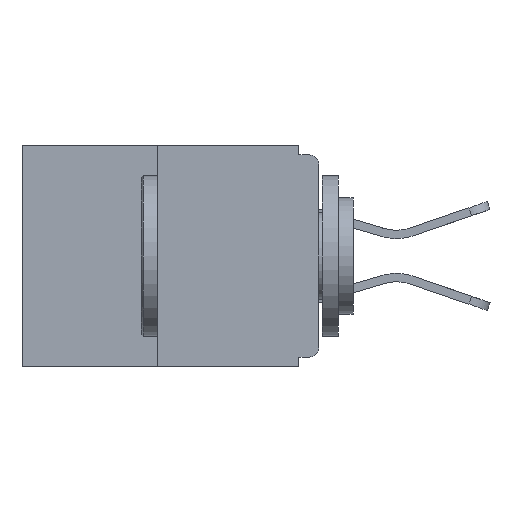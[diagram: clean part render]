
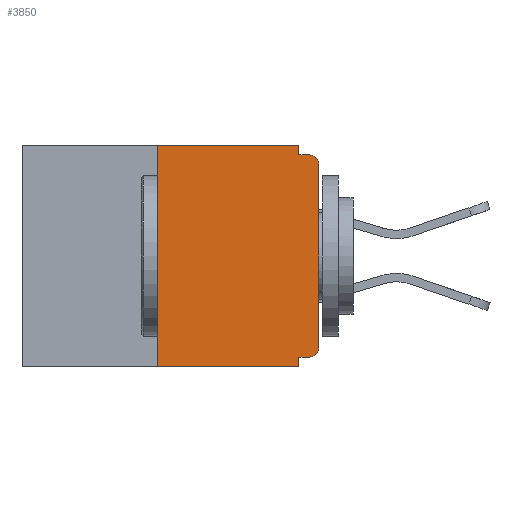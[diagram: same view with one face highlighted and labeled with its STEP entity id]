
A CAD part, left-side view. The second image highlights one B-rep face of the part: STEP entity #3850.
In plain terms, the highlighted planar face has unit normal (-1, 0, 0).
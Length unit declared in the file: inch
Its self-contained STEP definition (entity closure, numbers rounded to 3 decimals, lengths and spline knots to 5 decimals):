
#227 = ORIENTED_EDGE ( 'NONE', *, *, #5894, .F. ) ;
#260 = LINE ( 'NONE', #735, #8915 ) ;
#568 = EDGE_CURVE ( 'NONE', #2424, #10036, #5878, .T. ) ;
#735 = CARTESIAN_POINT ( 'NONE',  ( 0., 0.46, -0.343 ) ) ;
#929 = VERTEX_POINT ( 'NONE', #13095 ) ;
#1142 = CARTESIAN_POINT ( 'NONE',  ( 0., 0., -0.313 ) ) ;
#1813 = CARTESIAN_POINT ( 'NONE',  ( 0., 0.031, -0.328 ) ) ;
#1955 = DIRECTION ( 'NONE',  ( 0., 0., 1. ) ) ;
#2094 = ORIENTED_EDGE ( 'NONE', *, *, #3684, .F. ) ;
#2167 = DIRECTION ( 'NONE',  ( -1., 0., 0. ) ) ;
#2347 = ORIENTED_EDGE ( 'NONE', *, *, #5990, .T. ) ;
#2424 = VERTEX_POINT ( 'NONE', #9496 ) ;
#2529 = VECTOR ( 'NONE', #4888, 39.37008 ) ;
#2824 = VECTOR ( 'NONE', #11935, 39.37008 ) ;
#3253 = VERTEX_POINT ( 'NONE', #1142 ) ;
#3391 = AXIS2_PLACEMENT_3D ( 'NONE', #13987, #2167, #11065 ) ;
#3684 = EDGE_CURVE ( 'NONE', #12927, #6191, #9129, .T. ) ;
#3850 = ADVANCED_FACE ( 'NONE', ( #4232 ), #11746, .F. ) ;
#4232 = FACE_OUTER_BOUND ( 'NONE', #18196, .T. ) ;
#4669 = AXIS2_PLACEMENT_3D ( 'NONE', #5122, #17075, #9638 ) ;
#4710 = CARTESIAN_POINT ( 'NONE',  ( 0., 0., -0.03 ) ) ;
#4888 = DIRECTION ( 'NONE',  ( 0., -1., 0. ) ) ;
#4936 = ORIENTED_EDGE ( 'NONE', *, *, #15292, .T. ) ;
#5122 = CARTESIAN_POINT ( 'NONE',  ( 0., 0.015, -0.03 ) ) ;
#5578 = CARTESIAN_POINT ( 'NONE',  ( 0., 0.031, -0.343 ) ) ;
#5813 = LINE ( 'NONE', #12353, #6223 ) ;
#5878 = LINE ( 'NONE', #9089, #8910 ) ;
#5894 = EDGE_CURVE ( 'NONE', #6191, #929, #8827, .T. ) ;
#5990 = EDGE_CURVE ( 'NONE', #3253, #8307, #5813, .T. ) ;
#6085 = CARTESIAN_POINT ( 'NONE',  ( 0., 0.25, -0.343 ) ) ;
#6191 = VERTEX_POINT ( 'NONE', #1813 ) ;
#6223 = VECTOR ( 'NONE', #1955, 39.37008 ) ;
#6483 = LINE ( 'NONE', #9465, #2529 ) ;
#6603 = EDGE_CURVE ( 'NONE', #10737, #2424, #6483, .T. ) ;
#6862 = DIRECTION ( 'NONE',  ( 0., -1., 0. ) ) ;
#7127 = LINE ( 'NONE', #11748, #9440 ) ;
#7496 = CARTESIAN_POINT ( 'NONE',  ( 0., 0.25, 0. ) ) ;
#7677 = EDGE_CURVE ( 'NONE', #10233, #10737, #7127, .T. ) ;
#7755 = VECTOR ( 'NONE', #9927, 39.37008 ) ;
#8307 = VERTEX_POINT ( 'NONE', #4710 ) ;
#8444 = CARTESIAN_POINT ( 'NONE',  ( 0., 0., -0.015 ) ) ;
#8827 = LINE ( 'NONE', #5578, #11625 ) ;
#8893 = ORIENTED_EDGE ( 'NONE', *, *, #18392, .T. ) ;
#8910 = VECTOR ( 'NONE', #16576, 39.37008 ) ;
#8915 = VECTOR ( 'NONE', #6862, 39.37008 ) ;
#9089 = CARTESIAN_POINT ( 'NONE',  ( 0., 0.031, 0. ) ) ;
#9129 = LINE ( 'NONE', #16234, #2824 ) ;
#9440 = VECTOR ( 'NONE', #19218, 39.37008 ) ;
#9465 = CARTESIAN_POINT ( 'NONE',  ( 0., 0.46, 0. ) ) ;
#9496 = CARTESIAN_POINT ( 'NONE',  ( 0., 0.031, 0. ) ) ;
#9638 = DIRECTION ( 'NONE',  ( 0., 0., -1. ) ) ;
#9644 = CARTESIAN_POINT ( 'NONE',  ( 0., 0.031, -0.015 ) ) ;
#9742 = CARTESIAN_POINT ( 'NONE',  ( 0., 0.015, -0.328 ) ) ;
#9927 = DIRECTION ( 'NONE',  ( 0., -1., 0. ) ) ;
#10036 = VERTEX_POINT ( 'NONE', #9644 ) ;
#10179 = DIRECTION ( 'NONE',  ( 0., 0., -1. ) ) ;
#10233 = VERTEX_POINT ( 'NONE', #6085 ) ;
#10299 = VERTEX_POINT ( 'NONE', #15488 ) ;
#10481 = ORIENTED_EDGE ( 'NONE', *, *, #18587, .F. ) ;
#10737 = VERTEX_POINT ( 'NONE', #7496 ) ;
#11065 = DIRECTION ( 'NONE',  ( 0., 0., -1. ) ) ;
#11625 = VECTOR ( 'NONE', #16008, 39.37008 ) ;
#11746 = PLANE ( 'NONE',  #16217 ) ;
#11748 = CARTESIAN_POINT ( 'NONE',  ( 0., 0.25, 0. ) ) ;
#11935 = DIRECTION ( 'NONE',  ( 0., 1., 0. ) ) ;
#12073 = CIRCLE ( 'NONE', #4669, 0.015 ) ;
#12353 = CARTESIAN_POINT ( 'NONE',  ( 0., 0., 0. ) ) ;
#12709 = ORIENTED_EDGE ( 'NONE', *, *, #7677, .F. ) ;
#12925 = EDGE_CURVE ( 'NONE', #12927, #3253, #18080, .T. ) ;
#12927 = VERTEX_POINT ( 'NONE', #9742 ) ;
#13095 = CARTESIAN_POINT ( 'NONE',  ( 0., 0.031, -0.343 ) ) ;
#13133 = LINE ( 'NONE', #8444, #7755 ) ;
#13987 = CARTESIAN_POINT ( 'NONE',  ( 0., 0.015, -0.313 ) ) ;
#15292 = EDGE_CURVE ( 'NONE', #8307, #10299, #12073, .T. ) ;
#15488 = CARTESIAN_POINT ( 'NONE',  ( 0., 0.015, -0.015 ) ) ;
#16008 = DIRECTION ( 'NONE',  ( 0., 0., -1. ) ) ;
#16217 = AXIS2_PLACEMENT_3D ( 'NONE', #17545, #18961, #10179 ) ;
#16234 = CARTESIAN_POINT ( 'NONE',  ( 0., 0., -0.328 ) ) ;
#16288 = ORIENTED_EDGE ( 'NONE', *, *, #12925, .T. ) ;
#16576 = DIRECTION ( 'NONE',  ( 0., 0., -1. ) ) ;
#17075 = DIRECTION ( 'NONE',  ( -1., 0., 0. ) ) ;
#17545 = CARTESIAN_POINT ( 'NONE',  ( 0., 0.46, 0. ) ) ;
#17716 = ORIENTED_EDGE ( 'NONE', *, *, #6603, .F. ) ;
#18080 = CIRCLE ( 'NONE', #3391, 0.015 ) ;
#18196 = EDGE_LOOP ( 'NONE', ( #17716, #12709, #8893, #227, #2094, #16288, #2347, #4936, #10481, #18975 ) ) ;
#18392 = EDGE_CURVE ( 'NONE', #10233, #929, #260, .T. ) ;
#18587 = EDGE_CURVE ( 'NONE', #10036, #10299, #13133, .T. ) ;
#18961 = DIRECTION ( 'NONE',  ( 1., 0., 0. ) ) ;
#18975 = ORIENTED_EDGE ( 'NONE', *, *, #568, .F. ) ;
#19218 = DIRECTION ( 'NONE',  ( 0., 0., 1. ) ) ;
